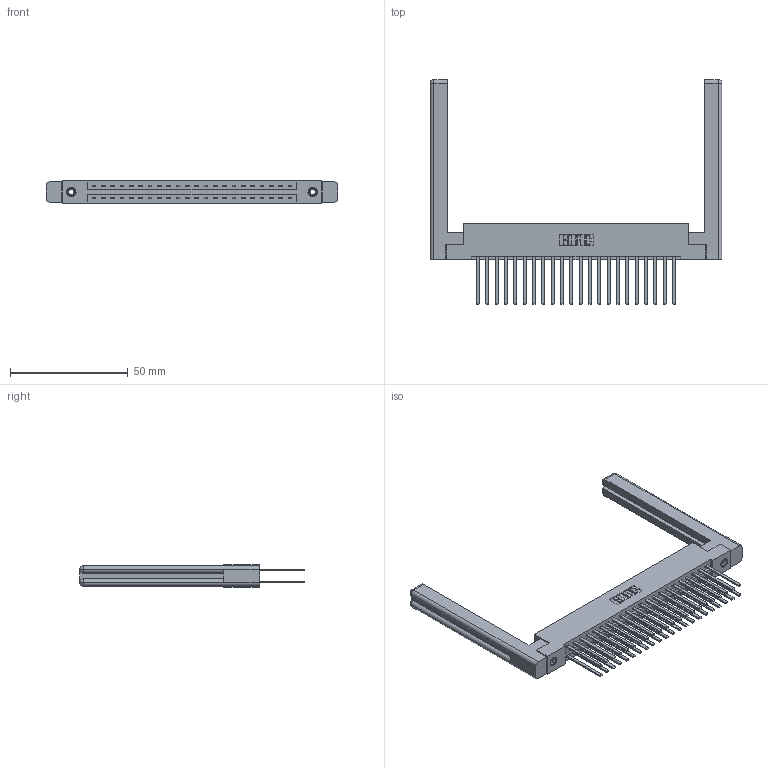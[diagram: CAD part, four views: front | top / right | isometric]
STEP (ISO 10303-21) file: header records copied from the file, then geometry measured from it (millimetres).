
FILE_DESCRIPTION (( 'STEP AP203' ), '1' );
FILE_NAME ('387-044-544-258.STEP', '2019-10-18T06:03:14', ( '' ), ( '' ), 'SwSTEP 2.0', 'SolidWorks 2016', '' );
FILE_SCHEMA (( 'CONFIG_CONTROL_DESIGN' ));
Length unit declared in the file: inch
Products named in the file (5): 307-220-058; 387-044-544-258; 345-292-001_345-293-144; 345-250-001_345-250-001-102; 337 Part_Flush Mounting Lugs - 0.156 Dia-TI
Assembly tree (49 placements, depth 2):
  387-044-544-258
    337 Part_Flush Mounting Lugs - 0.156 Dia-TI
    345-292-001_345-293-144  x44
    345-250-001_345-250-001-102  x2
    307-220-058  x2
Bounding box: 123.8 x 95.38 x 9.4 mm (x, y, z)
Volume: 20539.9 mm3; surface area: 22013.4 mm2
Topology: 49 solids, 49 shells, 2368 faces, 6957 edges, 4566 vertices
Faces by surface type: plane 1650, cylinder 694, cone 12, torus 12
Entity records: 22094 total; most frequent: CARTESIAN_POINT 3745, ORIENTED_EDGE 3620, DIRECTION 3234, EDGE_CURVE 1810, VECTOR 1638, LINE 1638, VERTEX_POINT 1198, AXIS2_PLACEMENT_3D 798
